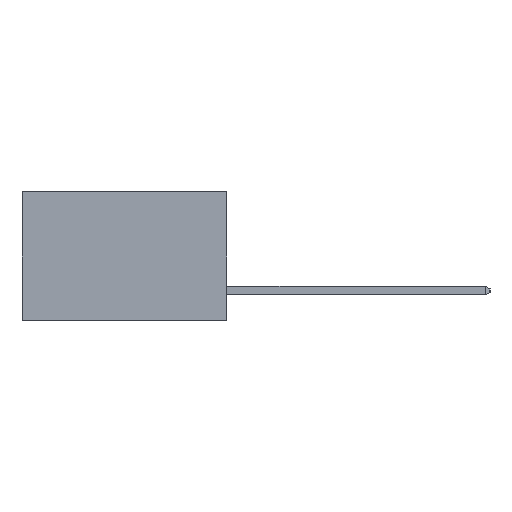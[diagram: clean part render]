
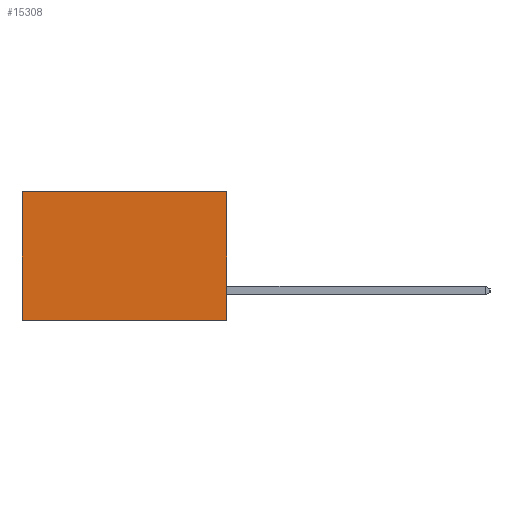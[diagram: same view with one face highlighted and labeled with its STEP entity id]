
A CAD part, left-side view. The second image highlights one B-rep face of the part: STEP entity #15308.
In plain terms, the highlighted planar face has unit normal (-1, 0, 0).
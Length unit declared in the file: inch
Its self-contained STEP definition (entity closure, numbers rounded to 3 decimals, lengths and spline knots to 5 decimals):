
#383 = PLANE ( 'NONE',  #20953 ) ;
#433 = VERTEX_POINT ( 'NONE', #26818 ) ;
#1727 = ORIENTED_EDGE ( 'NONE', *, *, #19352, .T. ) ;
#2964 = CARTESIAN_POINT ( 'NONE',  ( 0.277, 0., -0.37 ) ) ;
#3897 = VERTEX_POINT ( 'NONE', #15821 ) ;
#4044 = DIRECTION ( 'NONE',  ( 0., 0., -1. ) ) ;
#4540 = DIRECTION ( 'NONE',  ( 0., 1., 0. ) ) ;
#4601 = CARTESIAN_POINT ( 'NONE',  ( 0.277, 0., -0.37 ) ) ;
#4640 = ORIENTED_EDGE ( 'NONE', *, *, #20832, .T. ) ;
#5571 = DIRECTION ( 'NONE',  ( 1., 0., 0. ) ) ;
#5913 = EDGE_LOOP ( 'NONE', ( #4640, #18376, #18804, #1727 ) ) ;
#9053 = CARTESIAN_POINT ( 'NONE',  ( 0.277, 0., -0.37 ) ) ;
#9066 = EDGE_CURVE ( 'NONE', #433, #17465, #28131, .T. ) ;
#10791 = CARTESIAN_POINT ( 'NONE',  ( 0.277, 0., 0. ) ) ;
#11039 = CARTESIAN_POINT ( 'NONE',  ( 0.277, 0., 0. ) ) ;
#11618 = DIRECTION ( 'NONE',  ( 0., 0., -1. ) ) ;
#11682 = CARTESIAN_POINT ( 'NONE',  ( 0.277, 0.59, -0.37 ) ) ;
#14956 = LINE ( 'NONE', #9053, #20810 ) ;
#15308 = ADVANCED_FACE ( 'NONE', ( #22572 ), #383, .F. ) ;
#15390 = VERTEX_POINT ( 'NONE', #10791 ) ;
#15821 = CARTESIAN_POINT ( 'NONE',  ( 0.277, 0.59, 0. ) ) ;
#16651 = LINE ( 'NONE', #11039, #29732 ) ;
#17465 = VERTEX_POINT ( 'NONE', #11682 ) ;
#17725 = LINE ( 'NONE', #19175, #31469 ) ;
#18376 = ORIENTED_EDGE ( 'NONE', *, *, #9066, .F. ) ;
#18804 = ORIENTED_EDGE ( 'NONE', *, *, #22243, .F. ) ;
#19175 = CARTESIAN_POINT ( 'NONE',  ( 0.277, 0.59, -0.37 ) ) ;
#19352 = EDGE_CURVE ( 'NONE', #15390, #3897, #16651, .T. ) ;
#20810 = VECTOR ( 'NONE', #11618, 39.37008 ) ;
#20832 = EDGE_CURVE ( 'NONE', #3897, #17465, #17725, .T. ) ;
#20953 = AXIS2_PLACEMENT_3D ( 'NONE', #2964, #5571, #23145 ) ;
#22243 = EDGE_CURVE ( 'NONE', #15390, #433, #14956, .T. ) ;
#22572 = FACE_OUTER_BOUND ( 'NONE', #5913, .T. ) ;
#23145 = DIRECTION ( 'NONE',  ( 0., 0., -1. ) ) ;
#26818 = CARTESIAN_POINT ( 'NONE',  ( 0.277, 0., -0.37 ) ) ;
#27361 = VECTOR ( 'NONE', #4540, 39.37008 ) ;
#28131 = LINE ( 'NONE', #4601, #27361 ) ;
#28405 = DIRECTION ( 'NONE',  ( 0., 1., 0. ) ) ;
#29732 = VECTOR ( 'NONE', #28405, 39.37008 ) ;
#31469 = VECTOR ( 'NONE', #4044, 39.37008 ) ;
